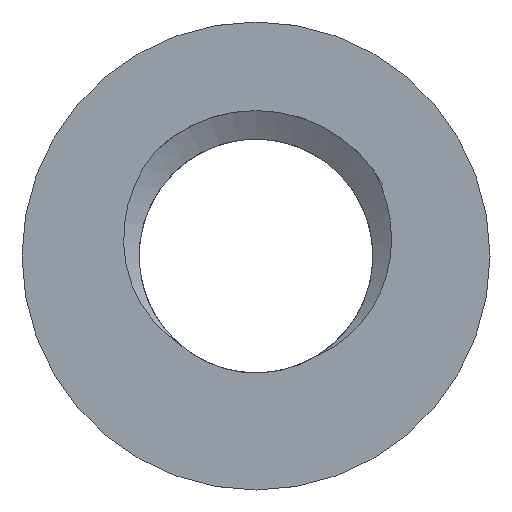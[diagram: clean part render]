
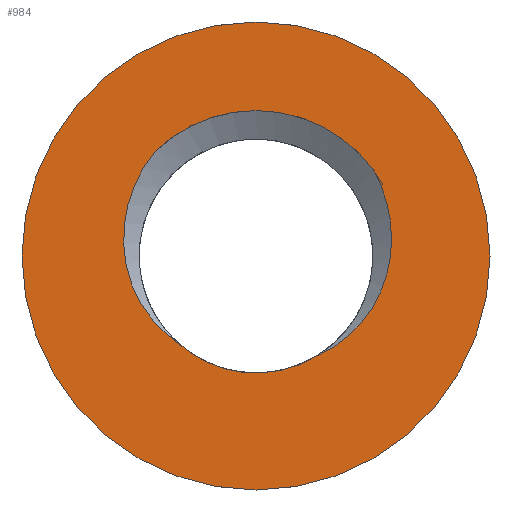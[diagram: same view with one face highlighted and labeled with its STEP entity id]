
A CAD part, front view. The second image highlights one B-rep face of the part: STEP entity #984.
In plain terms, the highlighted planar face has unit normal (0, -1, 0).
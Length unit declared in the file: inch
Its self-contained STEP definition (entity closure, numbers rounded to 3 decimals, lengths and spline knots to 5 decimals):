
#26 = AXIS2_PLACEMENT_3D ( 'NONE', #1533, #396, #688 ) ;
#28 = CARTESIAN_POINT ( 'NONE',  ( 0.25, 0., 2.815 ) ) ;
#38 = CARTESIAN_POINT ( 'NONE',  ( 0.28115, 0., 2.61238 ) ) ;
#62 = CARTESIAN_POINT ( 'NONE',  ( 0.25, 0., 2.7 ) ) ;
#109 = CARTESIAN_POINT ( 'NONE',  ( 0.16631, 0., 2.778 ) ) ;
#124 = CARTESIAN_POINT ( 'NONE',  ( 0.14822, 0., 2.73939 ) ) ;
#139 = VERTEX_POINT ( 'NONE', #28 ) ;
#140 = CARTESIAN_POINT ( 'NONE',  ( 0.17603, 0., 2.64081 ) ) ;
#146 = CARTESIAN_POINT ( 'NONE',  ( 0.15254, 0., 2.75304 ) ) ;
#147 = CARTESIAN_POINT ( 'NONE',  ( 0.19109, 0., 2.62857 ) ) ;
#160 = CARTESIAN_POINT ( 'NONE',  ( 0.22181, 0., 2.61181 ) ) ;
#212 = CARTESIAN_POINT ( 'NONE',  ( 0.35723, 0., 2.71968 ) ) ;
#215 = DIRECTION ( 'NONE',  ( 0., 1., 0. ) ) ;
#224 = PLANE ( 'NONE',  #322 ) ;
#225 = DIRECTION ( 'NONE',  ( 0., 0., 1. ) ) ;
#263 = CIRCLE ( 'NONE', #531, 0.115 ) ;
#293 = EDGE_CURVE ( 'NONE', #1620, #913, #1731, .T. ) ;
#310 = CARTESIAN_POINT ( 'NONE',  ( 0.20795, 0., 2.61752 ) ) ;
#321 = DIRECTION ( 'NONE',  ( 0., 0., 1. ) ) ;
#322 = AXIS2_PLACEMENT_3D ( 'NONE', #62, #215, #483 ) ;
#339 = CARTESIAN_POINT ( 'NONE',  ( 0.26652, 0., 2.6089 ) ) ;
#359 = CARTESIAN_POINT ( 'NONE',  ( 0.3433, 0., 2.76723 ) ) ;
#383 = EDGE_CURVE ( 'NONE', #540, #139, #263, .T. ) ;
#396 = DIRECTION ( 'NONE',  ( 0., 1., 0. ) ) ;
#474 = CARTESIAN_POINT ( 'NONE',  ( 0.29047, 0., 2.61627 ) ) ;
#477 = CARTESIAN_POINT ( 'NONE',  ( 0.34678, 0., 2.76094 ) ) ;
#483 = DIRECTION ( 'NONE',  ( 0., 0., 1. ) ) ;
#484 = DIRECTION ( 'NONE',  ( 0., 0., 1. ) ) ;
#486 = CARTESIAN_POINT ( 'NONE',  ( 0.3485, 0., 2.67099 ) ) ;
#531 = AXIS2_PLACEMENT_3D ( 'NONE', #1053, #1204, #225 ) ;
#540 = VERTEX_POINT ( 'NONE', #1060 ) ;
#549 = CARTESIAN_POINT ( 'NONE',  ( 0.15203, 0., 2.67614 ) ) ;
#569 = CARTESIAN_POINT ( 'NONE',  ( 0.15493, 0., 2.66954 ) ) ;
#573 = EDGE_CURVE ( 'NONE', #1284, #1210, #1144, .T. ) ;
#578 = CARTESIAN_POINT ( 'NONE',  ( 0.2465, 0., 2.60748 ) ) ;
#586 = ORIENTED_EDGE ( 'NONE', *, *, #383, .T. ) ;
#653 = CIRCLE ( 'NONE', #26, 0.185 ) ;
#667 = FACE_OUTER_BOUND ( 'NONE', #1550, .T. ) ;
#688 = DIRECTION ( 'NONE',  ( 0., 0., 1. ) ) ;
#711 = ORIENTED_EDGE ( 'NONE', *, *, #573, .F. ) ;
#715 = CARTESIAN_POINT ( 'NONE',  ( 0.18737, 0., 2.632 ) ) ;
#737 = CARTESIAN_POINT ( 'NONE',  ( 0.31179, 0., 2.6281 ) ) ;
#740 = CARTESIAN_POINT ( 'NONE',  ( 0.19506, 0., 2.62548 ) ) ;
#751 = CARTESIAN_POINT ( 'NONE',  ( 0.25, 0., 2.515 ) ) ;
#759 = AXIS2_PLACEMENT_3D ( 'NONE', #1491, #1335, #484 ) ;
#763 = CARTESIAN_POINT ( 'NONE',  ( 0.35636, 0., 2.69837 ) ) ;
#766 = CARTESIAN_POINT ( 'NONE',  ( 0.32842, 0., 2.64168 ) ) ;
#795 = CARTESIAN_POINT ( 'NONE',  ( 0.3433, 0., 2.76723 ) ) ;
#801 = ORIENTED_EDGE ( 'NONE', *, *, #1243, .F. ) ;
#806 = EDGE_CURVE ( 'NONE', #1113, #1284, #1401, .T. ) ;
#818 = CARTESIAN_POINT ( 'NONE',  ( 0.1554, 0., 2.75969 ) ) ;
#834 = B_SPLINE_CURVE_WITH_KNOTS ( 'NONE', 3,
 ( #1095, #109, #1676, #818, #146, #124, #1438, #1711, #1269, #1288, #1833, #549, #569, #1839, #1139, #140, #1692, #856 ),
 .UNSPECIFIED., .F., .F.,
 ( 4, 2, 2, 2, 2, 2, 2, 2, 4 ),
 ( 0., 0.00054, 0.00108, 0.00162, 0.00217, 0.00271, 0.00325, 0.00379, 0.00433 ),
 .UNSPECIFIED. ) ;
#856 = CARTESIAN_POINT ( 'NONE',  ( 0.18737, 0., 2.632 ) ) ;
#858 = CARTESIAN_POINT ( 'NONE',  ( 0.2171, 0., 2.61346 ) ) ;
#909 = CARTESIAN_POINT ( 'NONE',  ( 0.34963, 0., 2.75433 ) ) ;
#913 = VERTEX_POINT ( 'NONE', #751 ) ;
#917 = CARTESIAN_POINT ( 'NONE',  ( 0.34174, 0., 2.65842 ) ) ;
#984 = ADVANCED_FACE ( 'NONE', ( #667, #1763 ), #224, .F. ) ;
#1007 = ORIENTED_EDGE ( 'NONE', *, *, #293, .F. ) ;
#1011 = CIRCLE ( 'NONE', #1553, 0.115 ) ;
#1032 = ORIENTED_EDGE ( 'NONE', *, *, #1446, .T. ) ;
#1033 = CARTESIAN_POINT ( 'NONE',  ( 0.29905, 0., 2.62164 ) ) ;
#1053 = CARTESIAN_POINT ( 'NONE',  ( 0.25, 0., 2.7 ) ) ;
#1060 = CARTESIAN_POINT ( 'NONE',  ( 0.17095, 0., 2.78352 ) ) ;
#1061 = CARTESIAN_POINT ( 'NONE',  ( 0.35552, 0., 2.7339 ) ) ;
#1064 = CARTESIAN_POINT ( 'NONE',  ( 0.35118, 0., 2.67755 ) ) ;
#1095 = CARTESIAN_POINT ( 'NONE',  ( 0.17095, 0., 2.78352 ) ) ;
#1113 = VERTEX_POINT ( 'NONE', #1228 ) ;
#1139 = CARTESIAN_POINT ( 'NONE',  ( 0.16631, 0., 2.65139 ) ) ;
#1144 = B_SPLINE_CURVE_WITH_KNOTS ( 'NONE', 3,
 ( #1481, #1621, #737, #1189, #766, #1640, #917, #486, #1064, #1338, #763, #1636, #212, #1061, #1777, #909, #477, #359 ),
 .UNSPECIFIED., .F., .F.,
 ( 4, 2, 2, 2, 2, 2, 2, 2, 4 ),
 ( 0., 0.00054, 0.00108, 0.00163, 0.00217, 0.00271, 0.00325, 0.00379, 0.00433 ),
 .UNSPECIFIED. ) ;
#1189 = CARTESIAN_POINT ( 'NONE',  ( 0.32316, 0., 2.63672 ) ) ;
#1204 = DIRECTION ( 'NONE',  ( 0., 1., 0. ) ) ;
#1210 = VERTEX_POINT ( 'NONE', #795 ) ;
#1226 = ORIENTED_EDGE ( 'NONE', *, *, #1332, .F. ) ;
#1228 = CARTESIAN_POINT ( 'NONE',  ( 0.18737, 0., 2.632 ) ) ;
#1243 = EDGE_CURVE ( 'NONE', #913, #1620, #653, .T. ) ;
#1269 = CARTESIAN_POINT ( 'NONE',  ( 0.14513, 0., 2.711 ) ) ;
#1284 = VERTEX_POINT ( 'NONE', #1403 ) ;
#1288 = CARTESIAN_POINT ( 'NONE',  ( 0.1464, 0., 2.69682 ) ) ;
#1289 = CARTESIAN_POINT ( 'NONE',  ( 0.23151, 0., 2.60928 ) ) ;
#1332 = EDGE_CURVE ( 'NONE', #540, #1113, #834, .T. ) ;
#1335 = DIRECTION ( 'NONE',  ( 0., 1., 0. ) ) ;
#1338 = CARTESIAN_POINT ( 'NONE',  ( 0.35513, 0., 2.69124 ) ) ;
#1401 = B_SPLINE_CURVE_WITH_KNOTS ( 'NONE', 3,
 ( #715, #147, #740, #1743, #310, #858, #160, #1289, #1447, #578, #1611, #1760, #339, #38, #474, #1033 ),
 .UNSPECIFIED., .F., .F.,
 ( 4, 2, 2, 2, 2, 2, 2, 4 ),
 ( 0., 0.00038, 0.00077, 0.00115, 0.00153, 0.00192, 0.0023, 0.00307 ),
 .UNSPECIFIED. ) ;
#1403 = CARTESIAN_POINT ( 'NONE',  ( 0.29905, 0., 2.62164 ) ) ;
#1438 = CARTESIAN_POINT ( 'NONE',  ( 0.14676, 0., 2.73244 ) ) ;
#1446 = EDGE_CURVE ( 'NONE', #139, #1210, #1011, .T. ) ;
#1447 = CARTESIAN_POINT ( 'NONE',  ( 0.23653, 0., 2.6084 ) ) ;
#1481 = CARTESIAN_POINT ( 'NONE',  ( 0.29905, 0., 2.62164 ) ) ;
#1491 = CARTESIAN_POINT ( 'NONE',  ( 0.25, 0., 2.7 ) ) ;
#1503 = ORIENTED_EDGE ( 'NONE', *, *, #806, .F. ) ;
#1511 = CARTESIAN_POINT ( 'NONE',  ( 0.25, 0., 2.885 ) ) ;
#1533 = CARTESIAN_POINT ( 'NONE',  ( 0.25, 0., 2.7 ) ) ;
#1550 = EDGE_LOOP ( 'NONE', ( #801, #1007 ) ) ;
#1553 = AXIS2_PLACEMENT_3D ( 'NONE', #1586, #1606, #321 ) ;
#1586 = CARTESIAN_POINT ( 'NONE',  ( 0.25, 0., 2.7 ) ) ;
#1606 = DIRECTION ( 'NONE',  ( 0., 1., 0. ) ) ;
#1611 = CARTESIAN_POINT ( 'NONE',  ( 0.25149, 0., 2.60743 ) ) ;
#1620 = VERTEX_POINT ( 'NONE', #1511 ) ;
#1621 = CARTESIAN_POINT ( 'NONE',  ( 0.30565, 0., 2.6245 ) ) ;
#1636 = CARTESIAN_POINT ( 'NONE',  ( 0.35739, 0., 2.71253 ) ) ;
#1640 = CARTESIAN_POINT ( 'NONE',  ( 0.33766, 0., 2.65247 ) ) ;
#1676 = CARTESIAN_POINT ( 'NONE',  ( 0.16227, 0., 2.77213 ) ) ;
#1692 = CARTESIAN_POINT ( 'NONE',  ( 0.18141, 0., 2.63609 ) ) ;
#1711 = CARTESIAN_POINT ( 'NONE',  ( 0.14521, 0., 2.71827 ) ) ;
#1731 = CIRCLE ( 'NONE', #759, 0.185 ) ;
#1743 = CARTESIAN_POINT ( 'NONE',  ( 0.20348, 0., 2.61995 ) ) ;
#1760 = CARTESIAN_POINT ( 'NONE',  ( 0.26148, 0., 2.60813 ) ) ;
#1763 = FACE_BOUND ( 'NONE', #1799, .T. ) ;
#1777 = CARTESIAN_POINT ( 'NONE',  ( 0.35399, 0., 2.74083 ) ) ;
#1799 = EDGE_LOOP ( 'NONE', ( #586, #1032, #711, #1503, #1226 ) ) ;
#1833 = CARTESIAN_POINT ( 'NONE',  ( 0.14774, 0., 2.68985 ) ) ;
#1839 = CARTESIAN_POINT ( 'NONE',  ( 0.16204, 0., 2.65722 ) ) ;
